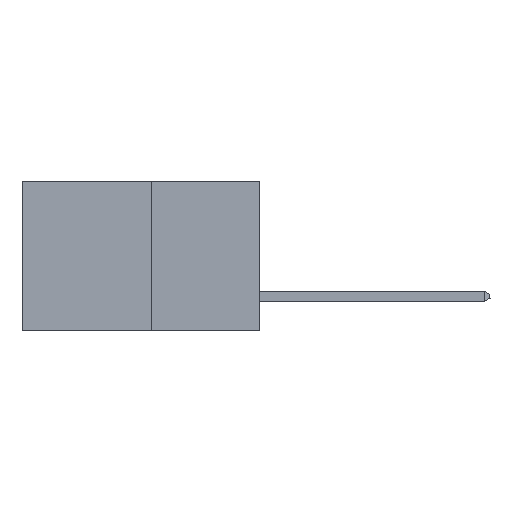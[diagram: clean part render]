
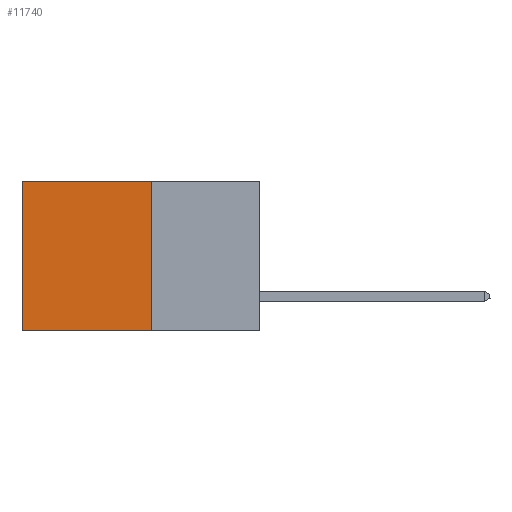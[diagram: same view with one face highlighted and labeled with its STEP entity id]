
A CAD part, left-side view. The second image highlights one B-rep face of the part: STEP entity #11740.
In plain terms, the highlighted planar face has unit normal (-1, 0, 0).
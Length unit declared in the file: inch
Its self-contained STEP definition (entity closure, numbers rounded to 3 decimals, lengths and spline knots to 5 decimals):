
#745 = CARTESIAN_POINT ( 'NONE',  ( 0.277, 0.27, 0. ) ) ;
#1879 = CARTESIAN_POINT ( 'NONE',  ( 0.277, 0.59, -0.37 ) ) ;
#1937 = VERTEX_POINT ( 'NONE', #24129 ) ;
#2301 = VERTEX_POINT ( 'NONE', #13029 ) ;
#3542 = DIRECTION ( 'NONE',  ( 0., 0., -1. ) ) ;
#5770 = LINE ( 'NONE', #15752, #25342 ) ;
#5830 = CARTESIAN_POINT ( 'NONE',  ( 0.277, 0.27, -0.37 ) ) ;
#7395 = CARTESIAN_POINT ( 'NONE',  ( 0.277, 0.27, 0. ) ) ;
#7896 = DIRECTION ( 'NONE',  ( 0., 0., -1. ) ) ;
#8165 = LINE ( 'NONE', #1879, #11734 ) ;
#8292 = VERTEX_POINT ( 'NONE', #7395 ) ;
#8864 = CARTESIAN_POINT ( 'NONE',  ( 0.277, 0.59, 0. ) ) ;
#11734 = VECTOR ( 'NONE', #20277, 39.37008 ) ;
#11740 = ADVANCED_FACE ( 'NONE', ( #24992 ), #18123, .F. ) ;
#12020 = LINE ( 'NONE', #745, #17441 ) ;
#13029 = CARTESIAN_POINT ( 'NONE',  ( 0.277, 0.59, -0.37 ) ) ;
#14629 = LINE ( 'NONE', #19338, #24593 ) ;
#15101 = EDGE_LOOP ( 'NONE', ( #20355, #20285, #21454, #25182 ) ) ;
#15752 = CARTESIAN_POINT ( 'NONE',  ( 0.277, 0.27, -0.37 ) ) ;
#17151 = DIRECTION ( 'NONE',  ( 0., 1., 0. ) ) ;
#17441 = VECTOR ( 'NONE', #17151, 39.37008 ) ;
#17996 = AXIS2_PLACEMENT_3D ( 'NONE', #5830, #20155, #7896 ) ;
#18123 = PLANE ( 'NONE',  #17996 ) ;
#19338 = CARTESIAN_POINT ( 'NONE',  ( 0.277, 0.27, -0.37 ) ) ;
#20155 = DIRECTION ( 'NONE',  ( 1., 0., 0. ) ) ;
#20277 = DIRECTION ( 'NONE',  ( 0., 0., -1. ) ) ;
#20285 = ORIENTED_EDGE ( 'NONE', *, *, #22747, .F. ) ;
#20355 = ORIENTED_EDGE ( 'NONE', *, *, #23055, .T. ) ;
#20694 = EDGE_CURVE ( 'NONE', #8292, #1937, #5770, .T. ) ;
#21323 = DIRECTION ( 'NONE',  ( 0., 1., 0. ) ) ;
#21454 = ORIENTED_EDGE ( 'NONE', *, *, #20694, .F. ) ;
#22747 = EDGE_CURVE ( 'NONE', #1937, #2301, #14629, .T. ) ;
#23055 = EDGE_CURVE ( 'NONE', #24534, #2301, #8165, .T. ) ;
#24129 = CARTESIAN_POINT ( 'NONE',  ( 0.277, 0.27, -0.37 ) ) ;
#24534 = VERTEX_POINT ( 'NONE', #8864 ) ;
#24593 = VECTOR ( 'NONE', #21323, 39.37008 ) ;
#24992 = FACE_OUTER_BOUND ( 'NONE', #15101, .T. ) ;
#25182 = ORIENTED_EDGE ( 'NONE', *, *, #25859, .T. ) ;
#25342 = VECTOR ( 'NONE', #3542, 39.37008 ) ;
#25859 = EDGE_CURVE ( 'NONE', #8292, #24534, #12020, .T. ) ;
